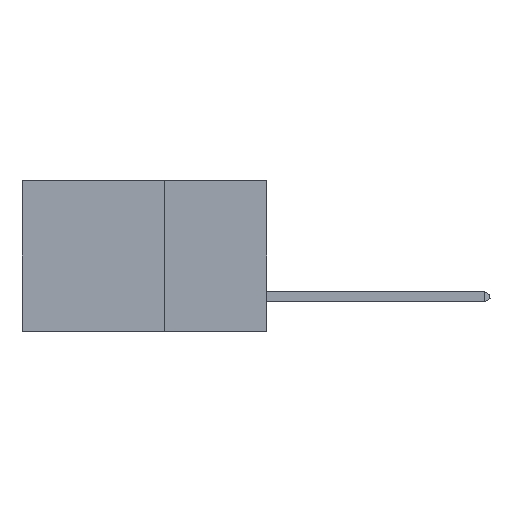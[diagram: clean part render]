
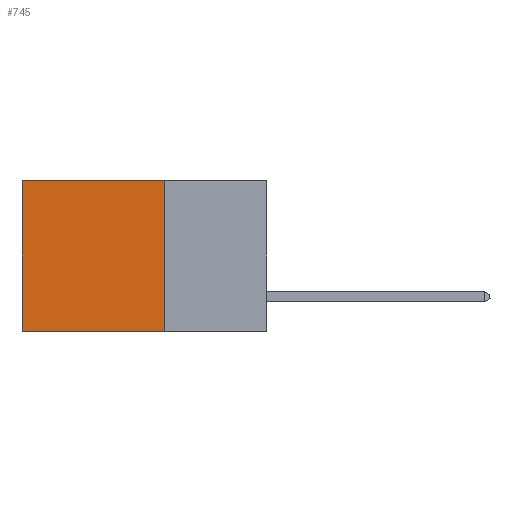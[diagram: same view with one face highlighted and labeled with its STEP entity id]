
A CAD part, left-side view. The second image highlights one B-rep face of the part: STEP entity #745.
In plain terms, the highlighted planar face has unit normal (-1, 0, 0).
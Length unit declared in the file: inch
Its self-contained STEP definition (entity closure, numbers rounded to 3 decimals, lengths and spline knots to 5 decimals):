
#745 = ADVANCED_FACE ( 'NONE', ( #13149 ), #15440, .F. ) ;
#968 = EDGE_CURVE ( 'NONE', #12355, #7840, #14295, .T. ) ;
#1053 = CARTESIAN_POINT ( 'NONE',  ( 0.2875, 0.25, 0. ) ) ;
#1148 = DIRECTION ( 'NONE',  ( 1., 0., 0. ) ) ;
#1331 = EDGE_LOOP ( 'NONE', ( #11738, #3912, #6093, #7752 ) ) ;
#1435 = AXIS2_PLACEMENT_3D ( 'NONE', #1053, #1148, #2047 ) ;
#1831 = CARTESIAN_POINT ( 'NONE',  ( 0.2875, 0.25, 0. ) ) ;
#1935 = CARTESIAN_POINT ( 'NONE',  ( 0.2875, 0.25, 0. ) ) ;
#2047 = DIRECTION ( 'NONE',  ( 0., 0., -1. ) ) ;
#2328 = LINE ( 'NONE', #15286, #15290 ) ;
#3912 = ORIENTED_EDGE ( 'NONE', *, *, #6159, .F. ) ;
#4084 = CARTESIAN_POINT ( 'NONE',  ( 0.2875, 0.25, -0.37 ) ) ;
#4110 = VECTOR ( 'NONE', #10196, 39.37008 ) ;
#4295 = EDGE_CURVE ( 'NONE', #12355, #13888, #6914, .T. ) ;
#6093 = ORIENTED_EDGE ( 'NONE', *, *, #4295, .F. ) ;
#6159 = EDGE_CURVE ( 'NONE', #13888, #12502, #2328, .T. ) ;
#6772 = VECTOR ( 'NONE', #11603, 39.37008 ) ;
#6914 = LINE ( 'NONE', #1935, #4110 ) ;
#7328 = LINE ( 'NONE', #9229, #8093 ) ;
#7752 = ORIENTED_EDGE ( 'NONE', *, *, #968, .T. ) ;
#7840 = VERTEX_POINT ( 'NONE', #8431 ) ;
#8093 = VECTOR ( 'NONE', #10269, 39.37008 ) ;
#8431 = CARTESIAN_POINT ( 'NONE',  ( 0.2875, 0.6, 0. ) ) ;
#9229 = CARTESIAN_POINT ( 'NONE',  ( 0.2875, 0.6, 0. ) ) ;
#9326 = DIRECTION ( 'NONE',  ( 0., 1., 0. ) ) ;
#9686 = CARTESIAN_POINT ( 'NONE',  ( 0.2875, 0.6, -0.37 ) ) ;
#10196 = DIRECTION ( 'NONE',  ( 0., 0., -1. ) ) ;
#10269 = DIRECTION ( 'NONE',  ( 0., 0., -1. ) ) ;
#11124 = EDGE_CURVE ( 'NONE', #7840, #12502, #7328, .T. ) ;
#11603 = DIRECTION ( 'NONE',  ( 0., 1., 0. ) ) ;
#11738 = ORIENTED_EDGE ( 'NONE', *, *, #11124, .T. ) ;
#12355 = VERTEX_POINT ( 'NONE', #13126 ) ;
#12502 = VERTEX_POINT ( 'NONE', #9686 ) ;
#13126 = CARTESIAN_POINT ( 'NONE',  ( 0.2875, 0.25, 0. ) ) ;
#13149 = FACE_OUTER_BOUND ( 'NONE', #1331, .T. ) ;
#13888 = VERTEX_POINT ( 'NONE', #4084 ) ;
#14295 = LINE ( 'NONE', #1831, #6772 ) ;
#15286 = CARTESIAN_POINT ( 'NONE',  ( 0.2875, 0.25, -0.37 ) ) ;
#15290 = VECTOR ( 'NONE', #9326, 39.37008 ) ;
#15440 = PLANE ( 'NONE',  #1435 ) ;
